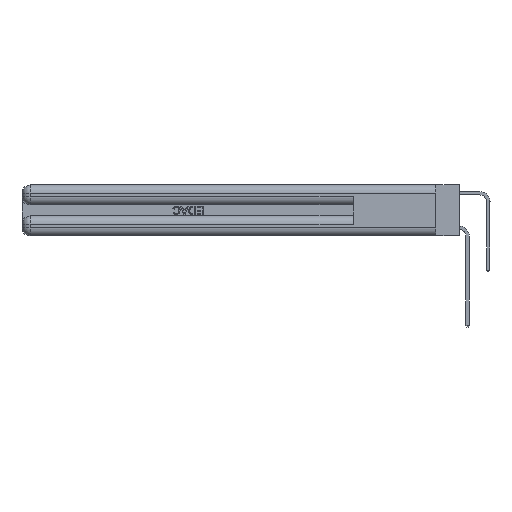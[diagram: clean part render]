
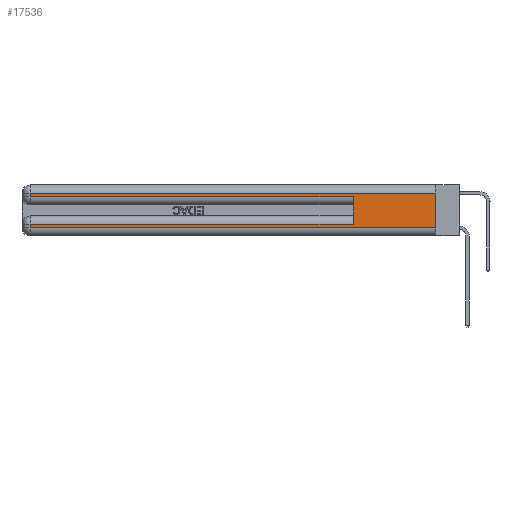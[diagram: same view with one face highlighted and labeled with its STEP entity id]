
A CAD part, left-side view. The second image highlights one B-rep face of the part: STEP entity #17536.
In plain terms, the highlighted planar face has unit normal (-1, 0, 0).
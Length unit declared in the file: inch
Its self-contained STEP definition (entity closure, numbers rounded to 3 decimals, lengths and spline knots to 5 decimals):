
#64 = CARTESIAN_POINT ( 'NONE',  ( 0., 2.94, 0.085 ) ) ;
#592 = CARTESIAN_POINT ( 'NONE',  ( 0., 0., 0.085 ) ) ;
#989 = LINE ( 'NONE', #38552, #23015 ) ;
#1482 = EDGE_CURVE ( 'NONE', #35777, #13895, #1668, .T. ) ;
#1668 = LINE ( 'NONE', #2299, #8218 ) ;
#2249 = VERTEX_POINT ( 'NONE', #6408 ) ;
#2299 = CARTESIAN_POINT ( 'NONE',  ( 0., 0.6, 0.145 ) ) ;
#2339 = PLANE ( 'NONE',  #10370 ) ;
#3692 = ORIENTED_EDGE ( 'NONE', *, *, #38327, .T. ) ;
#3815 = VECTOR ( 'NONE', #31255, 39.37008 ) ;
#3869 = VECTOR ( 'NONE', #7734, 39.37008 ) ;
#3956 = CARTESIAN_POINT ( 'NONE',  ( 0., 0., 0.285 ) ) ;
#4006 = CARTESIAN_POINT ( 'NONE',  ( 0., 2.94, 0.37 ) ) ;
#4334 = CARTESIAN_POINT ( 'NONE',  ( 0., 0., 0.31 ) ) ;
#4703 = LINE ( 'NONE', #7405, #27611 ) ;
#5204 = ORIENTED_EDGE ( 'NONE', *, *, #36230, .T. ) ;
#6408 = CARTESIAN_POINT ( 'NONE',  ( 0., 2.94, 0.31 ) ) ;
#7405 = CARTESIAN_POINT ( 'NONE',  ( 0., 0., 0.06 ) ) ;
#7734 = DIRECTION ( 'NONE',  ( 0., 0., -1. ) ) ;
#8218 = VECTOR ( 'NONE', #14958, 39.37008 ) ;
#10077 = CARTESIAN_POINT ( 'NONE',  ( 0., 0., 0.31 ) ) ;
#10298 = DIRECTION ( 'NONE',  ( 0., 1., 0. ) ) ;
#10322 = LINE ( 'NONE', #3956, #29061 ) ;
#10370 = AXIS2_PLACEMENT_3D ( 'NONE', #17351, #26386, #11513 ) ;
#10430 = LINE ( 'NONE', #13608, #3869 ) ;
#10981 = EDGE_LOOP ( 'NONE', ( #12870, #5204, #27078, #13641, #27399, #3692, #30563, #18134 ) ) ;
#11513 = DIRECTION ( 'NONE',  ( 0., 0., -1. ) ) ;
#12870 = ORIENTED_EDGE ( 'NONE', *, *, #16604, .F. ) ;
#13509 = CARTESIAN_POINT ( 'NONE',  ( 0., 0.6, 0.085 ) ) ;
#13608 = CARTESIAN_POINT ( 'NONE',  ( 0., 0., 0.37 ) ) ;
#13641 = ORIENTED_EDGE ( 'NONE', *, *, #20587, .T. ) ;
#13854 = EDGE_CURVE ( 'NONE', #23548, #35791, #36644, .T. ) ;
#13895 = VERTEX_POINT ( 'NONE', #16871 ) ;
#14958 = DIRECTION ( 'NONE',  ( 0., 0., 1. ) ) ;
#15260 = VERTEX_POINT ( 'NONE', #38636 ) ;
#16580 = VERTEX_POINT ( 'NONE', #22517 ) ;
#16604 = EDGE_CURVE ( 'NONE', #31317, #16580, #10430, .T. ) ;
#16610 = FACE_OUTER_BOUND ( 'NONE', #10981, .T. ) ;
#16871 = CARTESIAN_POINT ( 'NONE',  ( 0., 0.6, 0.285 ) ) ;
#17351 = CARTESIAN_POINT ( 'NONE',  ( 0., 0., 0.37 ) ) ;
#17536 = ADVANCED_FACE ( 'NONE', ( #16610 ), #2339, .F. ) ;
#18134 = ORIENTED_EDGE ( 'NONE', *, *, #30868, .T. ) ;
#18943 = DIRECTION ( 'NONE',  ( 0., -1., 0. ) ) ;
#19368 = DIRECTION ( 'NONE',  ( 0., 0., -1. ) ) ;
#20587 = EDGE_CURVE ( 'NONE', #15260, #13895, #10322, .T. ) ;
#20649 = DIRECTION ( 'NONE',  ( 0., 0., -1. ) ) ;
#21714 = VECTOR ( 'NONE', #10298, 39.37008 ) ;
#22517 = CARTESIAN_POINT ( 'NONE',  ( 0., 0., 0.06 ) ) ;
#23015 = VECTOR ( 'NONE', #20649, 39.37008 ) ;
#23548 = VERTEX_POINT ( 'NONE', #64 ) ;
#23616 = LINE ( 'NONE', #592, #21714 ) ;
#24887 = DIRECTION ( 'NONE',  ( 0., -1., 0. ) ) ;
#26386 = DIRECTION ( 'NONE',  ( 1., 0., 0. ) ) ;
#27078 = ORIENTED_EDGE ( 'NONE', *, *, #36534, .T. ) ;
#27399 = ORIENTED_EDGE ( 'NONE', *, *, #1482, .F. ) ;
#27611 = VECTOR ( 'NONE', #24887, 39.37008 ) ;
#28752 = VECTOR ( 'NONE', #19368, 39.37008 ) ;
#29061 = VECTOR ( 'NONE', #18943, 39.37008 ) ;
#30563 = ORIENTED_EDGE ( 'NONE', *, *, #13854, .T. ) ;
#30868 = EDGE_CURVE ( 'NONE', #35791, #16580, #4703, .T. ) ;
#31255 = DIRECTION ( 'NONE',  ( 0., 1., 0. ) ) ;
#31317 = VERTEX_POINT ( 'NONE', #10077 ) ;
#34553 = CARTESIAN_POINT ( 'NONE',  ( 0., 2.94, 0.06 ) ) ;
#35777 = VERTEX_POINT ( 'NONE', #13509 ) ;
#35791 = VERTEX_POINT ( 'NONE', #34553 ) ;
#36230 = EDGE_CURVE ( 'NONE', #31317, #2249, #37471, .T. ) ;
#36534 = EDGE_CURVE ( 'NONE', #2249, #15260, #989, .T. ) ;
#36644 = LINE ( 'NONE', #4006, #28752 ) ;
#37471 = LINE ( 'NONE', #4334, #3815 ) ;
#38327 = EDGE_CURVE ( 'NONE', #35777, #23548, #23616, .T. ) ;
#38552 = CARTESIAN_POINT ( 'NONE',  ( 0., 2.94, 0.37 ) ) ;
#38636 = CARTESIAN_POINT ( 'NONE',  ( 0., 2.94, 0.285 ) ) ;
